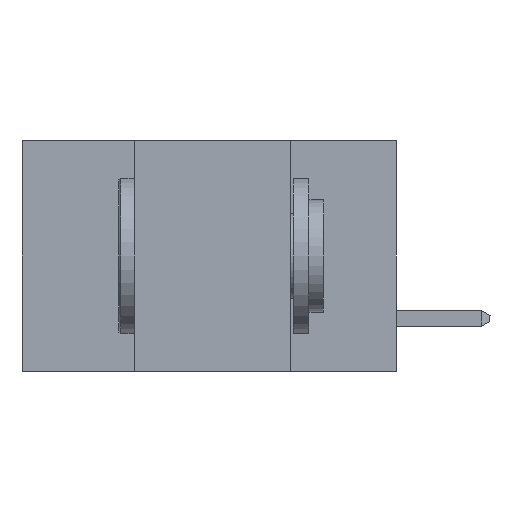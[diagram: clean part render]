
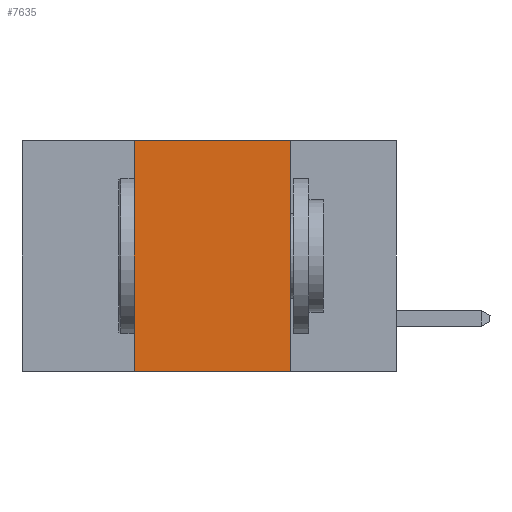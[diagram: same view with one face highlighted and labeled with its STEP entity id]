
A CAD part, left-side view. The second image highlights one B-rep face of the part: STEP entity #7635.
In plain terms, the highlighted planar face has unit normal (-1, 0, 0).
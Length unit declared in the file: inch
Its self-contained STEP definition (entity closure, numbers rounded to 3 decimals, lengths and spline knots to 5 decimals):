
#411 = CARTESIAN_POINT ( 'NONE',  ( 0., 0.42, 0. ) ) ;
#947 = ORIENTED_EDGE ( 'NONE', *, *, #20742, .F. ) ;
#1954 = DIRECTION ( 'NONE',  ( 0., -1., 0. ) ) ;
#2261 = ORIENTED_EDGE ( 'NONE', *, *, #17798, .F. ) ;
#2388 = CARTESIAN_POINT ( 'NONE',  ( 0., 0.6, 0. ) ) ;
#3679 = CARTESIAN_POINT ( 'NONE',  ( 0., 0.17, -0.37 ) ) ;
#4548 = EDGE_CURVE ( 'NONE', #19239, #7015, #9405, .T. ) ;
#6069 = VECTOR ( 'NONE', #10541, 39.37008 ) ;
#6583 = CARTESIAN_POINT ( 'NONE',  ( 0., 0.17, -0.37 ) ) ;
#6763 = DIRECTION ( 'NONE',  ( 0., 0., 1. ) ) ;
#7015 = VERTEX_POINT ( 'NONE', #3679 ) ;
#7469 = CARTESIAN_POINT ( 'NONE',  ( 0., 0.42, -0.37 ) ) ;
#7635 = ADVANCED_FACE ( 'NONE', ( #20111 ), #13933, .F. ) ;
#8822 = VERTEX_POINT ( 'NONE', #411 ) ;
#8949 = ORIENTED_EDGE ( 'NONE', *, *, #4548, .T. ) ;
#9263 = VERTEX_POINT ( 'NONE', #10650 ) ;
#9405 = LINE ( 'NONE', #19068, #10867 ) ;
#9948 = DIRECTION ( 'NONE',  ( 0., -1., 0. ) ) ;
#10541 = DIRECTION ( 'NONE',  ( 0., 0., -1. ) ) ;
#10650 = CARTESIAN_POINT ( 'NONE',  ( 0., 0.17, 0. ) ) ;
#10867 = VECTOR ( 'NONE', #1954, 39.37008 ) ;
#11327 = ORIENTED_EDGE ( 'NONE', *, *, #23051, .F. ) ;
#12146 = EDGE_LOOP ( 'NONE', ( #947, #2261, #11327, #8949 ) ) ;
#13574 = DIRECTION ( 'NONE',  ( 0., 0., -1. ) ) ;
#13933 = PLANE ( 'NONE',  #16660 ) ;
#14435 = LINE ( 'NONE', #18161, #14863 ) ;
#14863 = VECTOR ( 'NONE', #6763, 39.37008 ) ;
#16660 = AXIS2_PLACEMENT_3D ( 'NONE', #21527, #17279, #13574 ) ;
#17279 = DIRECTION ( 'NONE',  ( 1., 0., 0. ) ) ;
#17503 = VECTOR ( 'NONE', #9948, 39.37008 ) ;
#17798 = EDGE_CURVE ( 'NONE', #8822, #9263, #21261, .T. ) ;
#18161 = CARTESIAN_POINT ( 'NONE',  ( 0., 0.42, -0.37 ) ) ;
#19068 = CARTESIAN_POINT ( 'NONE',  ( 0., 0.6, -0.37 ) ) ;
#19239 = VERTEX_POINT ( 'NONE', #7469 ) ;
#20111 = FACE_OUTER_BOUND ( 'NONE', #12146, .T. ) ;
#20742 = EDGE_CURVE ( 'NONE', #9263, #7015, #23367, .T. ) ;
#21261 = LINE ( 'NONE', #2388, #17503 ) ;
#21527 = CARTESIAN_POINT ( 'NONE',  ( 0., 0.6, 0. ) ) ;
#23051 = EDGE_CURVE ( 'NONE', #19239, #8822, #14435, .T. ) ;
#23367 = LINE ( 'NONE', #6583, #6069 ) ;
